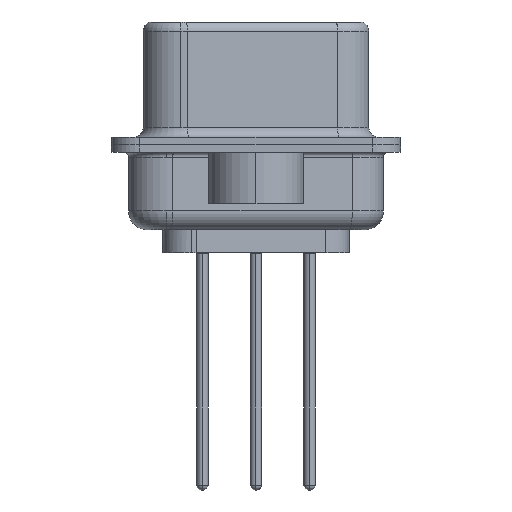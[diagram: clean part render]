
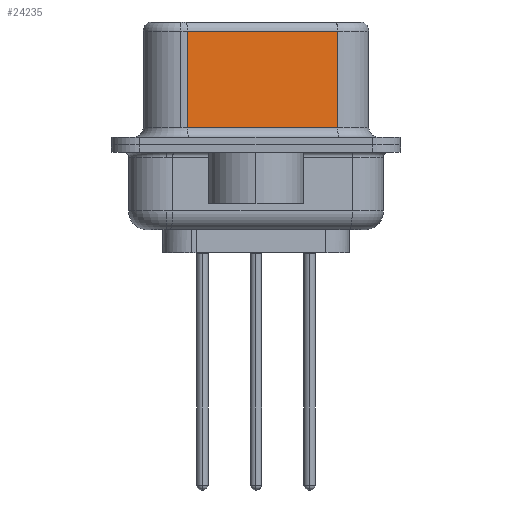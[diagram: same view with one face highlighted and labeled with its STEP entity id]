
A CAD part, left-side view. The second image highlights one B-rep face of the part: STEP entity #24235.
In plain terms, the highlighted planar face has unit normal (-0.985, -0.174, 0).
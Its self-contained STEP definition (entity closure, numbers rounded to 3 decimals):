
#2486 = CARTESIAN_POINT ( 'NONE',  ( 5.132, -4.322, 6.52 ) ) ;
#3028 = CARTESIAN_POINT ( 'NONE',  ( 3.73, 3.628, 0.9 ) ) ;
#3149 = VECTOR ( 'NONE', #16537, 1000. ) ;
#3608 = AXIS2_PLACEMENT_3D ( 'NONE', #2486, #4727, #27544 ) ;
#4727 = DIRECTION ( 'NONE',  ( 0.985, 0.174, 0. ) ) ;
#5384 = CARTESIAN_POINT ( 'NONE',  ( 5.132, -4.322, 0.9 ) ) ;
#5421 = CARTESIAN_POINT ( 'NONE',  ( 5.132, -4.322, 6.02 ) ) ;
#5538 = LINE ( 'NONE', #5384, #21177 ) ;
#6335 = LINE ( 'NONE', #15363, #11347 ) ;
#6568 = LINE ( 'NONE', #14194, #11920 ) ;
#7455 = VERTEX_POINT ( 'NONE', #5421 ) ;
#7936 = CARTESIAN_POINT ( 'NONE',  ( 3.73, 3.628, 6.52 ) ) ;
#8511 = VERTEX_POINT ( 'NONE', #11512 ) ;
#8784 = EDGE_CURVE ( 'NONE', #7455, #8511, #6335, .T. ) ;
#9020 = EDGE_CURVE ( 'NONE', #8511, #19106, #23649, .T. ) ;
#9781 = EDGE_CURVE ( 'NONE', #7455, #27625, #6568, .T. ) ;
#10992 = DIRECTION ( 'NONE',  ( 0., 0., -1. ) ) ;
#11347 = VECTOR ( 'NONE', #24404, 1000. ) ;
#11512 = CARTESIAN_POINT ( 'NONE',  ( 3.73, 3.628, 6.02 ) ) ;
#11920 = VECTOR ( 'NONE', #10992, 1000. ) ;
#14194 = CARTESIAN_POINT ( 'NONE',  ( 5.132, -4.322, 6.52 ) ) ;
#15363 = CARTESIAN_POINT ( 'NONE',  ( 5.132, -4.322, 6.02 ) ) ;
#16537 = DIRECTION ( 'NONE',  ( 0., 0., -1. ) ) ;
#16665 = EDGE_LOOP ( 'NONE', ( #19267, #22059, #21169, #24521 ) ) ;
#17235 = DIRECTION ( 'NONE',  ( 0.174, -0.985, 0. ) ) ;
#19106 = VERTEX_POINT ( 'NONE', #3028 ) ;
#19267 = ORIENTED_EDGE ( 'NONE', *, *, #9781, .F. ) ;
#21147 = PLANE ( 'NONE',  #3608 ) ;
#21169 = ORIENTED_EDGE ( 'NONE', *, *, #9020, .T. ) ;
#21177 = VECTOR ( 'NONE', #17235, 1000. ) ;
#22059 = ORIENTED_EDGE ( 'NONE', *, *, #8784, .T. ) ;
#23649 = LINE ( 'NONE', #7936, #3149 ) ;
#24235 = ADVANCED_FACE ( 'NONE', ( #25310 ), #21147, .F. ) ;
#24404 = DIRECTION ( 'NONE',  ( -0.174, 0.985, 0. ) ) ;
#24521 = ORIENTED_EDGE ( 'NONE', *, *, #27096, .T. ) ;
#25310 = FACE_OUTER_BOUND ( 'NONE', #16665, .T. ) ;
#27096 = EDGE_CURVE ( 'NONE', #19106, #27625, #5538, .T. ) ;
#27544 = DIRECTION ( 'NONE',  ( -0.174, 0.985, 0. ) ) ;
#27625 = VERTEX_POINT ( 'NONE', #29029 ) ;
#29029 = CARTESIAN_POINT ( 'NONE',  ( 5.132, -4.322, 0.9 ) ) ;
